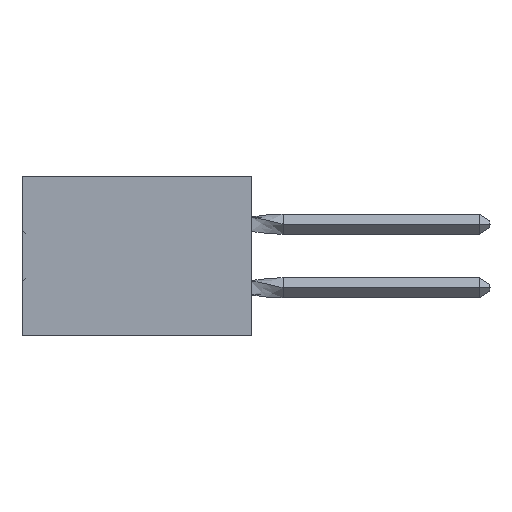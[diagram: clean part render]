
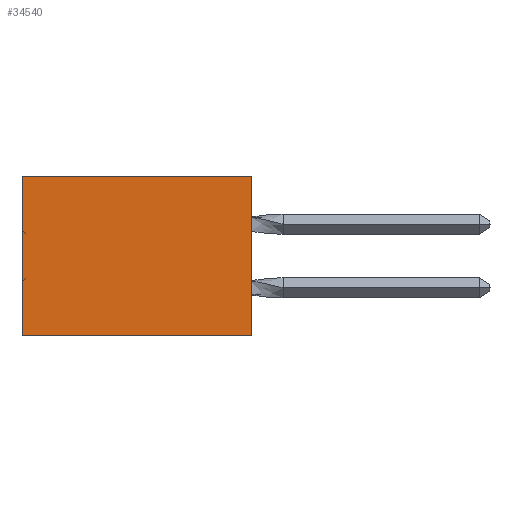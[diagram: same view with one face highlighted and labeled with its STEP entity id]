
A CAD part, left-side view. The second image highlights one B-rep face of the part: STEP entity #34540.
In plain terms, the highlighted planar face has unit normal (-1, 0, 0).
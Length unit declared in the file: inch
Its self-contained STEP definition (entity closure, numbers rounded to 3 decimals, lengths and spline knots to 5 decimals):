
#540 = FACE_OUTER_BOUND ( 'NONE', #60606, .T. ) ;
#1028 = PLANE ( 'NONE',  #34211 ) ;
#3900 = EDGE_CURVE ( 'NONE', #33308, #45417, #57476, .T. ) ;
#5830 = VECTOR ( 'NONE', #41196, 39.37008 ) ;
#6156 = CARTESIAN_POINT ( 'NONE',  ( 0.305, 0., -0.5 ) ) ;
#8453 = VECTOR ( 'NONE', #31474, 39.37008 ) ;
#9254 = EDGE_CURVE ( 'NONE', #30147, #45417, #31395, .T. ) ;
#10032 = DIRECTION ( 'NONE',  ( 0., 0., -1. ) ) ;
#10170 = DIRECTION ( 'NONE',  ( 0., 0., -1. ) ) ;
#11340 = ORIENTED_EDGE ( 'NONE', *, *, #24539, .T. ) ;
#11446 = LINE ( 'NONE', #60513, #29726 ) ;
#14559 = ORIENTED_EDGE ( 'NONE', *, *, #9254, .F. ) ;
#15538 = DIRECTION ( 'NONE',  ( 1., 0., 0. ) ) ;
#16602 = ORIENTED_EDGE ( 'NONE', *, *, #17374, .F. ) ;
#17374 = EDGE_CURVE ( 'NONE', #57982, #30147, #11446, .T. ) ;
#18237 = CARTESIAN_POINT ( 'NONE',  ( 0.305, 0., 0. ) ) ;
#18509 = VECTOR ( 'NONE', #22936, 39.37008 ) ;
#20010 = CARTESIAN_POINT ( 'NONE',  ( 0.305, 0., -0.5 ) ) ;
#22936 = DIRECTION ( 'NONE',  ( 0., 1., 0. ) ) ;
#24539 = EDGE_CURVE ( 'NONE', #57982, #33308, #34562, .T. ) ;
#29622 = CARTESIAN_POINT ( 'NONE',  ( 0.305, 0., 0. ) ) ;
#29726 = VECTOR ( 'NONE', #10170, 39.37008 ) ;
#30147 = VERTEX_POINT ( 'NONE', #20010 ) ;
#31270 = CARTESIAN_POINT ( 'NONE',  ( 0.305, 0.72, -0.5 ) ) ;
#31395 = LINE ( 'NONE', #59814, #5830 ) ;
#31474 = DIRECTION ( 'NONE',  ( 0., 0., -1. ) ) ;
#33308 = VERTEX_POINT ( 'NONE', #43140 ) ;
#34211 = AXIS2_PLACEMENT_3D ( 'NONE', #6156, #15538, #10032 ) ;
#34540 = ADVANCED_FACE ( 'NONE', ( #540 ), #1028, .F. ) ;
#34562 = LINE ( 'NONE', #18237, #18509 ) ;
#37200 = CARTESIAN_POINT ( 'NONE',  ( 0.305, 0.72, -0.5 ) ) ;
#41196 = DIRECTION ( 'NONE',  ( 0., 1., 0. ) ) ;
#43140 = CARTESIAN_POINT ( 'NONE',  ( 0.305, 0.72, 0. ) ) ;
#44760 = ORIENTED_EDGE ( 'NONE', *, *, #3900, .T. ) ;
#45417 = VERTEX_POINT ( 'NONE', #37200 ) ;
#57476 = LINE ( 'NONE', #31270, #8453 ) ;
#57982 = VERTEX_POINT ( 'NONE', #29622 ) ;
#59814 = CARTESIAN_POINT ( 'NONE',  ( 0.305, 0., -0.5 ) ) ;
#60513 = CARTESIAN_POINT ( 'NONE',  ( 0.305, 0., -0.5 ) ) ;
#60606 = EDGE_LOOP ( 'NONE', ( #44760, #14559, #16602, #11340 ) ) ;
